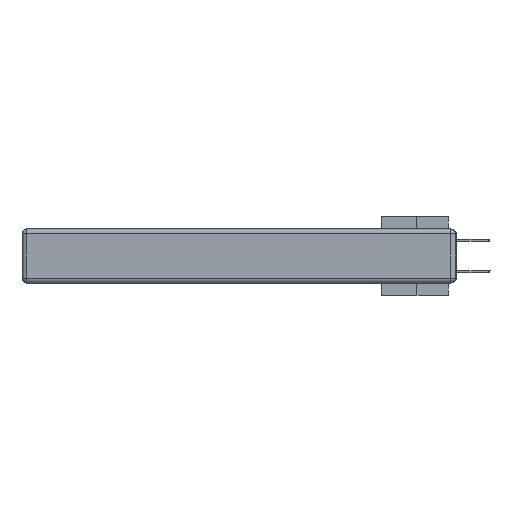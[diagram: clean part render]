
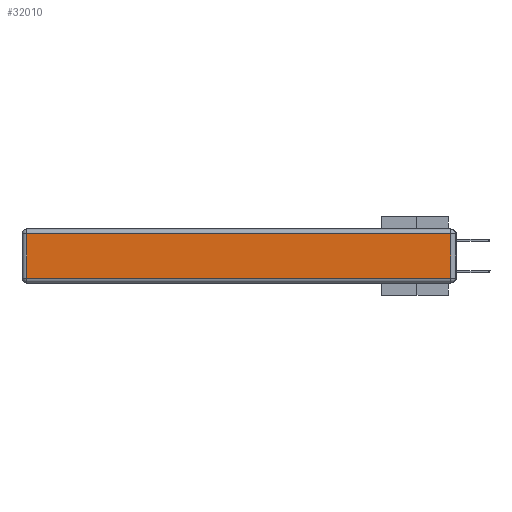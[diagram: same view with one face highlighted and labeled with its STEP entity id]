
A CAD part, left-side view. The second image highlights one B-rep face of the part: STEP entity #32010.
In plain terms, the highlighted planar face has unit normal (-1, 0, 0).
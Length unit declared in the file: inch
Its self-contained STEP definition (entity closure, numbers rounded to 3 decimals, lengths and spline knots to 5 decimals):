
#1219 = VERTEX_POINT ( 'NONE', #23327 ) ;
#2168 = ORIENTED_EDGE ( 'NONE', *, *, #14522, .T. ) ;
#3360 = EDGE_CURVE ( 'NONE', #18950, #1219, #24982, .T. ) ;
#4905 = ORIENTED_EDGE ( 'NONE', *, *, #26423, .T. ) ;
#5358 = ORIENTED_EDGE ( 'NONE', *, *, #32511, .T. ) ;
#6885 = ORIENTED_EDGE ( 'NONE', *, *, #3360, .T. ) ;
#7696 = LINE ( 'NONE', #19564, #33707 ) ;
#10369 = CARTESIAN_POINT ( 'NONE',  ( 0., 2.75, -0.03 ) ) ;
#11711 = LINE ( 'NONE', #26700, #23821 ) ;
#13554 = DIRECTION ( 'NONE',  ( -1., 0., 0. ) ) ;
#14328 = DIRECTION ( 'NONE',  ( 0., 0., 1. ) ) ;
#14522 = EDGE_CURVE ( 'NONE', #1219, #32628, #7696, .T. ) ;
#14585 = AXIS2_PLACEMENT_3D ( 'NONE', #31902, #13554, #14328 ) ;
#18950 = VERTEX_POINT ( 'NONE', #32295 ) ;
#19313 = DIRECTION ( 'NONE',  ( 0., 1., 0. ) ) ;
#19564 = CARTESIAN_POINT ( 'NONE',  ( 0., 2.72, -0.343 ) ) ;
#20347 = PLANE ( 'NONE',  #14585 ) ;
#21581 = VERTEX_POINT ( 'NONE', #23146 ) ;
#23146 = CARTESIAN_POINT ( 'NONE',  ( 0., 0.03, -0.313 ) ) ;
#23327 = CARTESIAN_POINT ( 'NONE',  ( 0., 2.72, -0.03 ) ) ;
#23821 = VECTOR ( 'NONE', #38260, 39.37008 ) ;
#24982 = LINE ( 'NONE', #10369, #31135 ) ;
#26423 = EDGE_CURVE ( 'NONE', #21581, #18950, #33719, .T. ) ;
#26700 = CARTESIAN_POINT ( 'NONE',  ( 0., 0., -0.313 ) ) ;
#27437 = CARTESIAN_POINT ( 'NONE',  ( 0., 0.03, -0.343 ) ) ;
#29379 = CARTESIAN_POINT ( 'NONE',  ( 0., 2.72, -0.313 ) ) ;
#31135 = VECTOR ( 'NONE', #19313, 39.37008 ) ;
#31495 = DIRECTION ( 'NONE',  ( 0., 0., -1. ) ) ;
#31902 = CARTESIAN_POINT ( 'NONE',  ( 0., 0., -0.343 ) ) ;
#32010 = ADVANCED_FACE ( 'NONE', ( #37969 ), #20347, .T. ) ;
#32295 = CARTESIAN_POINT ( 'NONE',  ( 0., 0.03, -0.03 ) ) ;
#32511 = EDGE_CURVE ( 'NONE', #32628, #21581, #11711, .T. ) ;
#32628 = VERTEX_POINT ( 'NONE', #29379 ) ;
#33090 = VECTOR ( 'NONE', #35880, 39.37008 ) ;
#33707 = VECTOR ( 'NONE', #31495, 39.37008 ) ;
#33719 = LINE ( 'NONE', #27437, #33090 ) ;
#35880 = DIRECTION ( 'NONE',  ( 0., 0., 1. ) ) ;
#37969 = FACE_OUTER_BOUND ( 'NONE', #38547, .T. ) ;
#38260 = DIRECTION ( 'NONE',  ( 0., -1., 0. ) ) ;
#38547 = EDGE_LOOP ( 'NONE', ( #5358, #4905, #6885, #2168 ) ) ;
